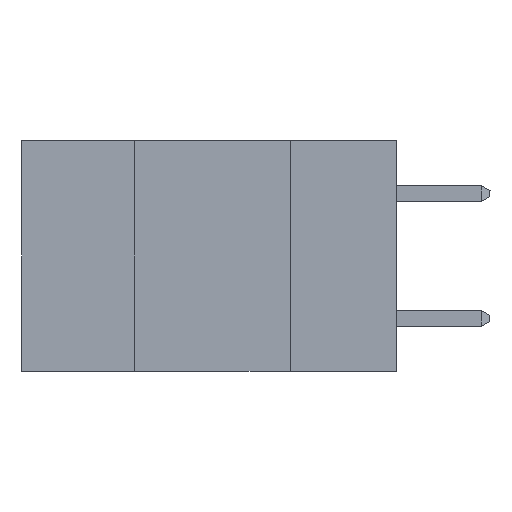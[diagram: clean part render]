
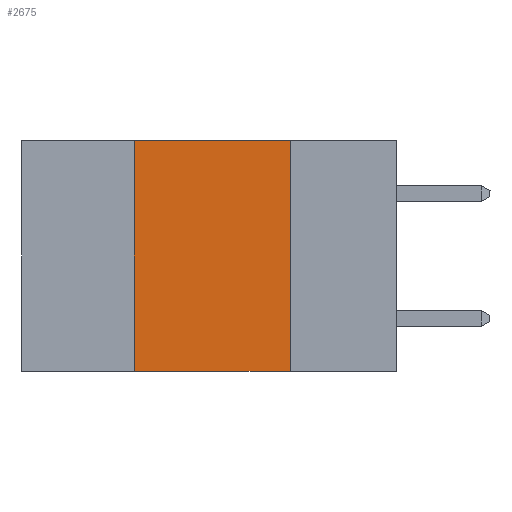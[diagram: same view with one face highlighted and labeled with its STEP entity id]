
A CAD part, left-side view. The second image highlights one B-rep face of the part: STEP entity #2675.
In plain terms, the highlighted planar face has unit normal (-1, 0, 0).
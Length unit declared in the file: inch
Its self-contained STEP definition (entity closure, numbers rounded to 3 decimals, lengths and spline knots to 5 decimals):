
#127 = VERTEX_POINT ( 'NONE', #1401 ) ;
#197 = VERTEX_POINT ( 'NONE', #1455 ) ;
#490 = ORIENTED_EDGE ( 'NONE', *, *, #1601, .F. ) ;
#822 = FACE_OUTER_BOUND ( 'NONE', #5629, .T. ) ;
#1401 = CARTESIAN_POINT ( 'NONE',  ( 0., 0.42, 0. ) ) ;
#1417 = VECTOR ( 'NONE', #2800, 39.37008 ) ;
#1455 = CARTESIAN_POINT ( 'NONE',  ( 0., 0.17, -0.37 ) ) ;
#1601 = EDGE_CURVE ( 'NONE', #8929, #127, #3234, .T. ) ;
#2551 = CARTESIAN_POINT ( 'NONE',  ( 0., 0.17, 0. ) ) ;
#2675 = ADVANCED_FACE ( 'NONE', ( #822 ), #8892, .F. ) ;
#2800 = DIRECTION ( 'NONE',  ( 0., 0., -1. ) ) ;
#3066 = CARTESIAN_POINT ( 'NONE',  ( 0., 0.6, 0. ) ) ;
#3177 = CARTESIAN_POINT ( 'NONE',  ( 0., 0.6, -0.37 ) ) ;
#3202 = ORIENTED_EDGE ( 'NONE', *, *, #6031, .F. ) ;
#3234 = LINE ( 'NONE', #6401, #3921 ) ;
#3270 = DIRECTION ( 'NONE',  ( 0., -1., 0. ) ) ;
#3476 = CARTESIAN_POINT ( 'NONE',  ( 0., 0.42, -0.37 ) ) ;
#3517 = VECTOR ( 'NONE', #7255, 39.37008 ) ;
#3530 = DIRECTION ( 'NONE',  ( 0., 0., -1. ) ) ;
#3532 = DIRECTION ( 'NONE',  ( 1., 0., 0. ) ) ;
#3921 = VECTOR ( 'NONE', #8987, 39.37008 ) ;
#4285 = EDGE_CURVE ( 'NONE', #127, #8840, #5218, .T. ) ;
#5129 = LINE ( 'NONE', #6722, #1417 ) ;
#5218 = LINE ( 'NONE', #8427, #3517 ) ;
#5540 = LINE ( 'NONE', #3177, #7499 ) ;
#5629 = EDGE_LOOP ( 'NONE', ( #3202, #8776, #490, #7095 ) ) ;
#6031 = EDGE_CURVE ( 'NONE', #8840, #197, #5129, .T. ) ;
#6401 = CARTESIAN_POINT ( 'NONE',  ( 0., 0.42, 0. ) ) ;
#6722 = CARTESIAN_POINT ( 'NONE',  ( 0., 0.17, 0. ) ) ;
#7095 = ORIENTED_EDGE ( 'NONE', *, *, #7320, .T. ) ;
#7255 = DIRECTION ( 'NONE',  ( 0., -1., 0. ) ) ;
#7320 = EDGE_CURVE ( 'NONE', #8929, #197, #5540, .T. ) ;
#7499 = VECTOR ( 'NONE', #3270, 39.37008 ) ;
#7574 = AXIS2_PLACEMENT_3D ( 'NONE', #3066, #3532, #3530 ) ;
#8427 = CARTESIAN_POINT ( 'NONE',  ( 0., 0.6, 0. ) ) ;
#8776 = ORIENTED_EDGE ( 'NONE', *, *, #4285, .F. ) ;
#8840 = VERTEX_POINT ( 'NONE', #2551 ) ;
#8892 = PLANE ( 'NONE',  #7574 ) ;
#8929 = VERTEX_POINT ( 'NONE', #3476 ) ;
#8987 = DIRECTION ( 'NONE',  ( 0., 0., 1. ) ) ;
